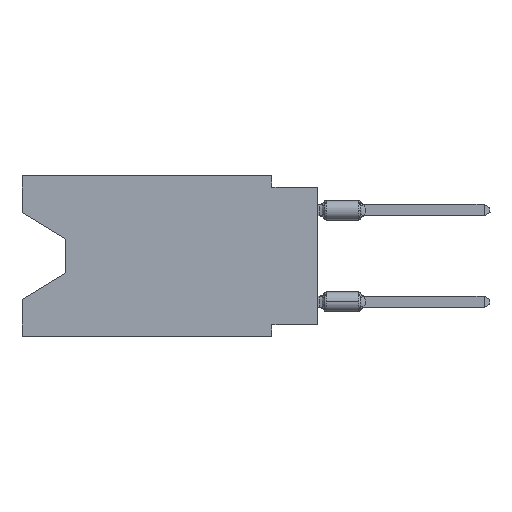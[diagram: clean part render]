
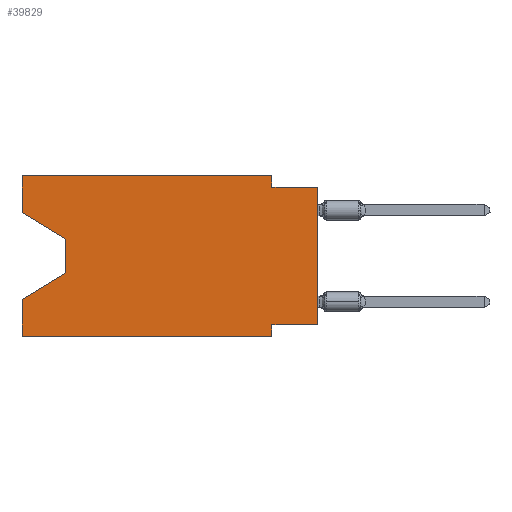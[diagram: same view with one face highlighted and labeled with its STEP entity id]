
A CAD part, left-side view. The second image highlights one B-rep face of the part: STEP entity #39829.
In plain terms, the highlighted planar face has unit normal (-1, 0, 0).
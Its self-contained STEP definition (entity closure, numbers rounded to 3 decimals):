
#868 = EDGE_LOOP ( 'NONE', ( #20058, #50297, #31550, #37239, #1003, #29581, #13551, #28890, #52040, #48400, #21532, #28554 ) ) ;
#1003 = ORIENTED_EDGE ( 'NONE', *, *, #42885, .T. ) ;
#1275 = LINE ( 'NONE', #49291, #47066 ) ;
#1952 = VERTEX_POINT ( 'NONE', #46686 ) ;
#2300 = VECTOR ( 'NONE', #4849, 1000. ) ;
#2390 = VERTEX_POINT ( 'NONE', #35791 ) ;
#2814 = CARTESIAN_POINT ( 'NONE',  ( 0., 16.383, 0. ) ) ;
#2884 = CARTESIAN_POINT ( 'NONE',  ( 0., 16.383, 0. ) ) ;
#3022 = CARTESIAN_POINT ( 'NONE',  ( 0., 16.383, -8.89 ) ) ;
#3889 = VECTOR ( 'NONE', #38569, 1000. ) ;
#4849 = DIRECTION ( 'NONE',  ( 0., 0., -1. ) ) ;
#5336 = LINE ( 'NONE', #45688, #44439 ) ;
#5629 = LINE ( 'NONE', #26211, #3889 ) ;
#5718 = DIRECTION ( 'NONE',  ( 0., 0., -1. ) ) ;
#5974 = VERTEX_POINT ( 'NONE', #38350 ) ;
#6034 = VECTOR ( 'NONE', #35844, 1000. ) ;
#7306 = DIRECTION ( 'NONE',  ( 0., 0., -1. ) ) ;
#7904 = EDGE_CURVE ( 'NONE', #21241, #21711, #50301, .T. ) ;
#8643 = EDGE_CURVE ( 'NONE', #32100, #18238, #5336, .T. ) ;
#10251 = LINE ( 'NONE', #22615, #11745 ) ;
#11745 = VECTOR ( 'NONE', #34216, 1000. ) ;
#12765 = CARTESIAN_POINT ( 'NONE',  ( 0., 13.97, -3.505 ) ) ;
#13510 = CARTESIAN_POINT ( 'NONE',  ( 0., 16.383, -2.038 ) ) ;
#13551 = ORIENTED_EDGE ( 'NONE', *, *, #35766, .F. ) ;
#13901 = AXIS2_PLACEMENT_3D ( 'NONE', #2814, #46856, #7306 ) ;
#14047 = DIRECTION ( 'NONE',  ( 0., 0., 1. ) ) ;
#14851 = VECTOR ( 'NONE', #40307, 1000. ) ;
#15811 = CARTESIAN_POINT ( 'NONE',  ( 0., 0., 0. ) ) ;
#16082 = CARTESIAN_POINT ( 'NONE',  ( 0., 2.54, -8.255 ) ) ;
#16851 = DIRECTION ( 'NONE',  ( 0., -1., 0. ) ) ;
#18238 = VERTEX_POINT ( 'NONE', #37484 ) ;
#19435 = CARTESIAN_POINT ( 'NONE',  ( 0., 0., -0.635 ) ) ;
#19886 = EDGE_CURVE ( 'NONE', #2390, #18238, #5629, .T. ) ;
#20058 = ORIENTED_EDGE ( 'NONE', *, *, #47972, .T. ) ;
#21241 = VERTEX_POINT ( 'NONE', #35152 ) ;
#21532 = ORIENTED_EDGE ( 'NONE', *, *, #34990, .F. ) ;
#21658 = VERTEX_POINT ( 'NONE', #13510 ) ;
#21711 = VERTEX_POINT ( 'NONE', #39030 ) ;
#21765 = LINE ( 'NONE', #37594, #49101 ) ;
#22615 = CARTESIAN_POINT ( 'NONE',  ( 0., 13.97, -3.505 ) ) ;
#22877 = FACE_OUTER_BOUND ( 'NONE', #868, .T. ) ;
#22981 = VECTOR ( 'NONE', #39535, 1000. ) ;
#23475 = CARTESIAN_POINT ( 'NONE',  ( 0., 0., -0.635 ) ) ;
#24010 = LINE ( 'NONE', #23475, #22981 ) ;
#25437 = LINE ( 'NONE', #49426, #41431 ) ;
#26211 = CARTESIAN_POINT ( 'NONE',  ( 0., 13.97, -5.385 ) ) ;
#27707 = CARTESIAN_POINT ( 'NONE',  ( 0., 16.383, -2.038 ) ) ;
#27953 = LINE ( 'NONE', #15811, #31592 ) ;
#28554 = ORIENTED_EDGE ( 'NONE', *, *, #33768, .F. ) ;
#28890 = ORIENTED_EDGE ( 'NONE', *, *, #39444, .T. ) ;
#29581 = ORIENTED_EDGE ( 'NONE', *, *, #49751, .F. ) ;
#30777 = PLANE ( 'NONE',  #13901 ) ;
#31109 = LINE ( 'NONE', #2884, #6034 ) ;
#31550 = ORIENTED_EDGE ( 'NONE', *, *, #19886, .T. ) ;
#31592 = VECTOR ( 'NONE', #31887, 1000. ) ;
#31887 = DIRECTION ( 'NONE',  ( 0., 0., 1. ) ) ;
#32100 = VERTEX_POINT ( 'NONE', #3022 ) ;
#33288 = VERTEX_POINT ( 'NONE', #12765 ) ;
#33768 = EDGE_CURVE ( 'NONE', #21658, #51159, #31109, .T. ) ;
#34216 = DIRECTION ( 'NONE',  ( 0., 0., -1. ) ) ;
#34990 = EDGE_CURVE ( 'NONE', #51159, #21241, #25437, .T. ) ;
#35152 = CARTESIAN_POINT ( 'NONE',  ( 0., 2.54, 0. ) ) ;
#35686 = EDGE_CURVE ( 'NONE', #21711, #42071, #24010, .T. ) ;
#35766 = EDGE_CURVE ( 'NONE', #1952, #46832, #21765, .T. ) ;
#35791 = CARTESIAN_POINT ( 'NONE',  ( 0., 13.97, -5.385 ) ) ;
#35844 = DIRECTION ( 'NONE',  ( 0., 0., 1. ) ) ;
#35851 = LINE ( 'NONE', #27707, #14851 ) ;
#35938 = CARTESIAN_POINT ( 'NONE',  ( 0., 16.383, 0. ) ) ;
#37239 = ORIENTED_EDGE ( 'NONE', *, *, #8643, .F. ) ;
#37484 = CARTESIAN_POINT ( 'NONE',  ( 0., 16.383, -6.852 ) ) ;
#37520 = DIRECTION ( 'NONE',  ( 0., -1., 0. ) ) ;
#37594 = CARTESIAN_POINT ( 'NONE',  ( 0., 0., -8.255 ) ) ;
#38350 = CARTESIAN_POINT ( 'NONE',  ( 0., 2.54, -8.89 ) ) ;
#38569 = DIRECTION ( 'NONE',  ( 0., 0.855, -0.519 ) ) ;
#39030 = CARTESIAN_POINT ( 'NONE',  ( 0., 2.54, -0.635 ) ) ;
#39444 = EDGE_CURVE ( 'NONE', #1952, #42071, #27953, .T. ) ;
#39535 = DIRECTION ( 'NONE',  ( 0., -1., 0. ) ) ;
#39829 = ADVANCED_FACE ( 'NONE', ( #22877 ), #30777, .F. ) ;
#40307 = DIRECTION ( 'NONE',  ( 0., -0.855, -0.519 ) ) ;
#41431 = VECTOR ( 'NONE', #37520, 1000. ) ;
#41735 = CARTESIAN_POINT ( 'NONE',  ( 0., 2.54, -8.89 ) ) ;
#41827 = CARTESIAN_POINT ( 'NONE',  ( 0., 2.54, 0. ) ) ;
#42071 = VERTEX_POINT ( 'NONE', #19435 ) ;
#42885 = EDGE_CURVE ( 'NONE', #32100, #5974, #1275, .T. ) ;
#43048 = EDGE_CURVE ( 'NONE', #33288, #2390, #10251, .T. ) ;
#44439 = VECTOR ( 'NONE', #14047, 1000. ) ;
#45688 = CARTESIAN_POINT ( 'NONE',  ( 0., 16.383, 0. ) ) ;
#45776 = DIRECTION ( 'NONE',  ( 0., 1., 0. ) ) ;
#46686 = CARTESIAN_POINT ( 'NONE',  ( 0., 0., -8.255 ) ) ;
#46832 = VERTEX_POINT ( 'NONE', #16082 ) ;
#46856 = DIRECTION ( 'NONE',  ( 1., 0., 0. ) ) ;
#47066 = VECTOR ( 'NONE', #16851, 1000. ) ;
#47972 = EDGE_CURVE ( 'NONE', #21658, #33288, #35851, .T. ) ;
#48400 = ORIENTED_EDGE ( 'NONE', *, *, #7904, .F. ) ;
#48653 = LINE ( 'NONE', #41735, #2300 ) ;
#49101 = VECTOR ( 'NONE', #45776, 1000. ) ;
#49291 = CARTESIAN_POINT ( 'NONE',  ( 0., 16.383, -8.89 ) ) ;
#49426 = CARTESIAN_POINT ( 'NONE',  ( 0., 16.383, 0. ) ) ;
#49751 = EDGE_CURVE ( 'NONE', #46832, #5974, #48653, .T. ) ;
#50297 = ORIENTED_EDGE ( 'NONE', *, *, #43048, .T. ) ;
#50301 = LINE ( 'NONE', #41827, #52048 ) ;
#51159 = VERTEX_POINT ( 'NONE', #35938 ) ;
#52040 = ORIENTED_EDGE ( 'NONE', *, *, #35686, .F. ) ;
#52048 = VECTOR ( 'NONE', #5718, 1000. ) ;
